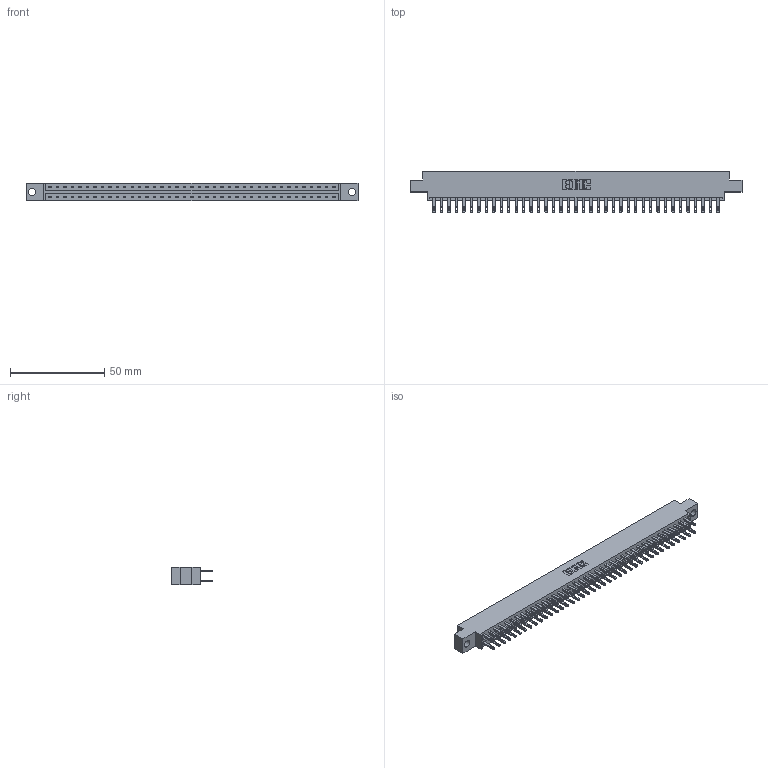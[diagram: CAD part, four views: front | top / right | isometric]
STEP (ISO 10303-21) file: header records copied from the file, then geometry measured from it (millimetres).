
FILE_DESCRIPTION (( 'STEP AP203' ), '1' );
FILE_NAME ('333-078-500-804.STEP', '2018-08-04T23:48:59', ( '' ), ( '' ), 'SwSTEP 2.0', 'SolidWorks 2016', '' );
FILE_SCHEMA (( 'CONFIG_CONTROL_DESIGN' ));
Length unit declared in the file: inch
Products named in the file (3): 333-078-500-804; 333 Part_Offset - .156 Dia - TH; 345-292-001_345-293-100
Assembly tree (79 placements, depth 2):
  333-078-500-804
    333 Part_Offset - .156 Dia - TH
    345-292-001_345-293-100  x78
Bounding box: 176.07 x 21.85 x 9.4 mm (x, y, z)
Volume: 17870.7 mm3; surface area: 21974 mm2
Topology: 79 solids, 79 shells, 3862 faces, 11789 edges, 7858 vertices
Faces by surface type: plane 2414, cylinder 1448
Entity records: 25543 total; most frequent: CARTESIAN_POINT 4238, ORIENTED_EDGE 4174, DIRECTION 3627, EDGE_CURVE 2087, LINE 1955, VECTOR 1955, VERTEX_POINT 1390, AXIS2_PLACEMENT_3D 836
